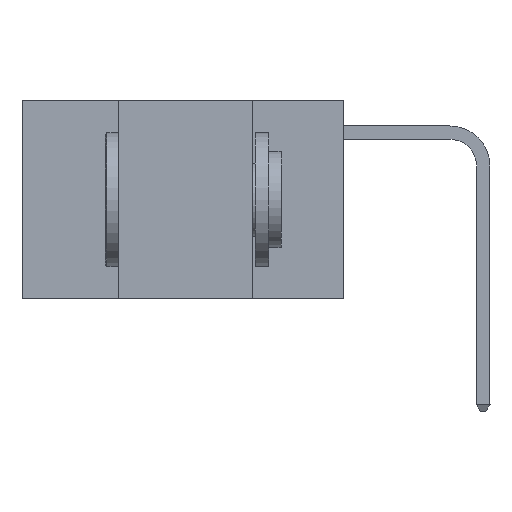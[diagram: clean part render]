
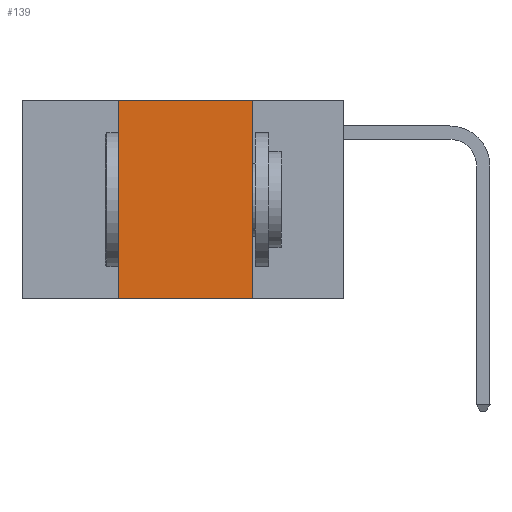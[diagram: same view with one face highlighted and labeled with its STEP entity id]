
A CAD part, left-side view. The second image highlights one B-rep face of the part: STEP entity #139.
In plain terms, the highlighted planar face has unit normal (-1, 0, 0).
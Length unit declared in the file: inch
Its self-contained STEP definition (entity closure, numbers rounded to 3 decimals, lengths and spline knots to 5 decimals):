
#139 = ADVANCED_FACE ( 'NONE', ( #8316 ), #19433, .F. ) ;
#2417 = EDGE_CURVE ( 'NONE', #7571, #11372, #17045, .T. ) ;
#3190 = CARTESIAN_POINT ( 'NONE',  ( 0., 0.6, -0.37 ) ) ;
#4310 = DIRECTION ( 'NONE',  ( 0., 0., 1. ) ) ;
#5424 = CARTESIAN_POINT ( 'NONE',  ( 0., 0.17, -0.37 ) ) ;
#5499 = DIRECTION ( 'NONE',  ( 0., -1., 0. ) ) ;
#5532 = LINE ( 'NONE', #3190, #27257 ) ;
#5973 = EDGE_CURVE ( 'NONE', #7289, #7571, #26986, .T. ) ;
#6284 = ORIENTED_EDGE ( 'NONE', *, *, #2417, .F. ) ;
#7289 = VERTEX_POINT ( 'NONE', #10946 ) ;
#7571 = VERTEX_POINT ( 'NONE', #20525 ) ;
#8316 = FACE_OUTER_BOUND ( 'NONE', #11411, .T. ) ;
#9243 = VECTOR ( 'NONE', #14126, 39.37008 ) ;
#10946 = CARTESIAN_POINT ( 'NONE',  ( 0., 0.42, -0.37 ) ) ;
#11372 = VERTEX_POINT ( 'NONE', #24063 ) ;
#11411 = EDGE_LOOP ( 'NONE', ( #17062, #6284, #24657, #22470 ) ) ;
#12612 = CARTESIAN_POINT ( 'NONE',  ( 0., 0.6, 0. ) ) ;
#12980 = VERTEX_POINT ( 'NONE', #5424 ) ;
#14126 = DIRECTION ( 'NONE',  ( 0., -1., 0. ) ) ;
#15288 = CARTESIAN_POINT ( 'NONE',  ( 0., 0.42, 0. ) ) ;
#15815 = VECTOR ( 'NONE', #23105, 39.37008 ) ;
#17045 = LINE ( 'NONE', #24919, #9243 ) ;
#17062 = ORIENTED_EDGE ( 'NONE', *, *, #20592, .F. ) ;
#17161 = LINE ( 'NONE', #27311, #15815 ) ;
#19433 = PLANE ( 'NONE',  #20252 ) ;
#20252 = AXIS2_PLACEMENT_3D ( 'NONE', #12612, #27409, #25476 ) ;
#20525 = CARTESIAN_POINT ( 'NONE',  ( 0., 0.42, 0. ) ) ;
#20592 = EDGE_CURVE ( 'NONE', #11372, #12980, #17161, .T. ) ;
#22470 = ORIENTED_EDGE ( 'NONE', *, *, #25473, .T. ) ;
#23105 = DIRECTION ( 'NONE',  ( 0., 0., -1. ) ) ;
#24063 = CARTESIAN_POINT ( 'NONE',  ( 0., 0.17, 0. ) ) ;
#24657 = ORIENTED_EDGE ( 'NONE', *, *, #5973, .F. ) ;
#24919 = CARTESIAN_POINT ( 'NONE',  ( 0., 0.6, 0. ) ) ;
#25473 = EDGE_CURVE ( 'NONE', #7289, #12980, #5532, .T. ) ;
#25476 = DIRECTION ( 'NONE',  ( 0., 0., -1. ) ) ;
#26986 = LINE ( 'NONE', #15288, #28305 ) ;
#27257 = VECTOR ( 'NONE', #5499, 39.37008 ) ;
#27311 = CARTESIAN_POINT ( 'NONE',  ( 0., 0.17, 0. ) ) ;
#27409 = DIRECTION ( 'NONE',  ( 1., 0., 0. ) ) ;
#28305 = VECTOR ( 'NONE', #4310, 39.37008 ) ;
